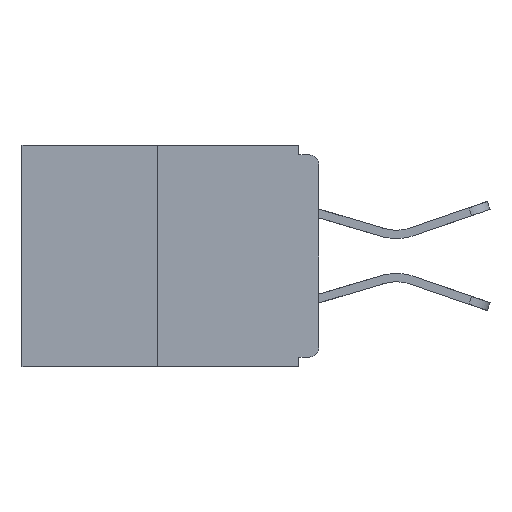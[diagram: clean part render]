
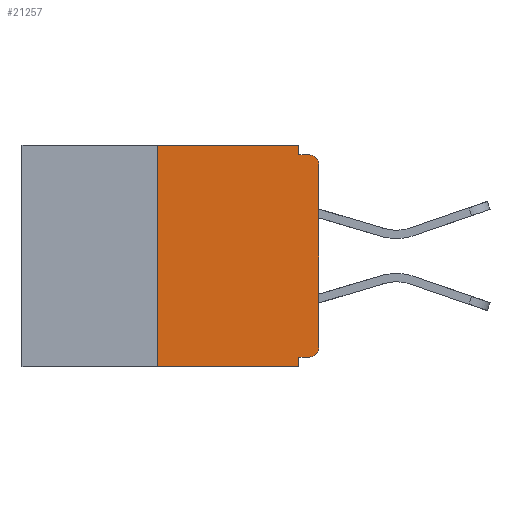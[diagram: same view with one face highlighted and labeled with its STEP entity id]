
A CAD part, left-side view. The second image highlights one B-rep face of the part: STEP entity #21257.
In plain terms, the highlighted planar face has unit normal (-1, 0, 0).
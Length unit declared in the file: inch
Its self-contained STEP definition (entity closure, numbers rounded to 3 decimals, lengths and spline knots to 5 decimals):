
#654 = CARTESIAN_POINT ( 'NONE',  ( 0., 0.031, 0. ) ) ;
#706 = DIRECTION ( 'NONE',  ( 0., 0., -1. ) ) ;
#2101 = CARTESIAN_POINT ( 'NONE',  ( 0., 0.25, -0.343 ) ) ;
#2222 = DIRECTION ( 'NONE',  ( 0., -1., 0. ) ) ;
#2345 = EDGE_LOOP ( 'NONE', ( #25715, #24356, #23364, #6456, #25840, #10254, #25453, #20279, #23910, #20800 ) ) ;
#2973 = CARTESIAN_POINT ( 'NONE',  ( 0., 0., 0. ) ) ;
#3060 = LINE ( 'NONE', #14448, #18005 ) ;
#3343 = CARTESIAN_POINT ( 'NONE',  ( 0., 0., -0.313 ) ) ;
#3421 = DIRECTION ( 'NONE',  ( -1., 0., 0. ) ) ;
#3853 = PLANE ( 'NONE',  #10965 ) ;
#4095 = FACE_OUTER_BOUND ( 'NONE', #2345, .T. ) ;
#4282 = CARTESIAN_POINT ( 'NONE',  ( 0., 0.015, -0.313 ) ) ;
#4431 = CARTESIAN_POINT ( 'NONE',  ( 0., 0., -0.328 ) ) ;
#4645 = CARTESIAN_POINT ( 'NONE',  ( 0., 0., -0.03 ) ) ;
#5353 = VERTEX_POINT ( 'NONE', #16338 ) ;
#6342 = DIRECTION ( 'NONE',  ( 0., 0., -1. ) ) ;
#6456 = ORIENTED_EDGE ( 'NONE', *, *, #26074, .F. ) ;
#6630 = CARTESIAN_POINT ( 'NONE',  ( 0., 0.46, -0.343 ) ) ;
#6662 = AXIS2_PLACEMENT_3D ( 'NONE', #15694, #3421, #9585 ) ;
#6745 = LINE ( 'NONE', #4431, #8318 ) ;
#6806 = VECTOR ( 'NONE', #12697, 39.37008 ) ;
#7884 = EDGE_CURVE ( 'NONE', #9522, #23636, #13813, .T. ) ;
#8318 = VECTOR ( 'NONE', #18672, 39.37008 ) ;
#8763 = CARTESIAN_POINT ( 'NONE',  ( 0., 0.015, -0.015 ) ) ;
#8769 = CARTESIAN_POINT ( 'NONE',  ( 0., 0.46, 0. ) ) ;
#9448 = CARTESIAN_POINT ( 'NONE',  ( 0., 0.031, -0.343 ) ) ;
#9522 = VERTEX_POINT ( 'NONE', #2101 ) ;
#9585 = DIRECTION ( 'NONE',  ( 0., 0., -1. ) ) ;
#9791 = EDGE_CURVE ( 'NONE', #18955, #23872, #25516, .T. ) ;
#9825 = DIRECTION ( 'NONE',  ( 0., 0., -1. ) ) ;
#9880 = EDGE_CURVE ( 'NONE', #17371, #15230, #22659, .T. ) ;
#10139 = LINE ( 'NONE', #17306, #19671 ) ;
#10254 = ORIENTED_EDGE ( 'NONE', *, *, #9880, .T. ) ;
#10605 = VERTEX_POINT ( 'NONE', #654 ) ;
#10965 = AXIS2_PLACEMENT_3D ( 'NONE', #15787, #22032, #19896 ) ;
#11363 = VERTEX_POINT ( 'NONE', #21166 ) ;
#11851 = VERTEX_POINT ( 'NONE', #20469 ) ;
#12511 = DIRECTION ( 'NONE',  ( -1., 0., 0. ) ) ;
#12588 = VECTOR ( 'NONE', #17211, 39.37008 ) ;
#12697 = DIRECTION ( 'NONE',  ( 0., -1., 0. ) ) ;
#13707 = LINE ( 'NONE', #13931, #24217 ) ;
#13813 = LINE ( 'NONE', #6630, #6806 ) ;
#13863 = LINE ( 'NONE', #2973, #12588 ) ;
#13931 = CARTESIAN_POINT ( 'NONE',  ( 0., 0.031, 0. ) ) ;
#14398 = LINE ( 'NONE', #25184, #21075 ) ;
#14448 = CARTESIAN_POINT ( 'NONE',  ( 0., 0., -0.015 ) ) ;
#15230 = VERTEX_POINT ( 'NONE', #3343 ) ;
#15578 = EDGE_CURVE ( 'NONE', #11363, #10605, #21980, .T. ) ;
#15694 = CARTESIAN_POINT ( 'NONE',  ( 0., 0.015, -0.03 ) ) ;
#15787 = CARTESIAN_POINT ( 'NONE',  ( 0., 0.46, 0. ) ) ;
#15808 = EDGE_CURVE ( 'NONE', #10605, #5353, #13707, .T. ) ;
#16338 = CARTESIAN_POINT ( 'NONE',  ( 0., 0.031, -0.015 ) ) ;
#16833 = DIRECTION ( 'NONE',  ( 0., -1., 0. ) ) ;
#17211 = DIRECTION ( 'NONE',  ( 0., 0., 1. ) ) ;
#17306 = CARTESIAN_POINT ( 'NONE',  ( 0., 0.25, 0. ) ) ;
#17371 = VERTEX_POINT ( 'NONE', #19542 ) ;
#17399 = AXIS2_PLACEMENT_3D ( 'NONE', #4282, #12511, #6342 ) ;
#17932 = EDGE_CURVE ( 'NONE', #15230, #18955, #13863, .T. ) ;
#18005 = VECTOR ( 'NONE', #2222, 39.37008 ) ;
#18672 = DIRECTION ( 'NONE',  ( 0., 1., 0. ) ) ;
#18955 = VERTEX_POINT ( 'NONE', #4645 ) ;
#19542 = CARTESIAN_POINT ( 'NONE',  ( 0., 0.015, -0.328 ) ) ;
#19671 = VECTOR ( 'NONE', #25588, 39.37008 ) ;
#19896 = DIRECTION ( 'NONE',  ( 0., 0., -1. ) ) ;
#20279 = ORIENTED_EDGE ( 'NONE', *, *, #9791, .T. ) ;
#20469 = CARTESIAN_POINT ( 'NONE',  ( 0., 0.031, -0.328 ) ) ;
#20800 = ORIENTED_EDGE ( 'NONE', *, *, #15808, .F. ) ;
#21075 = VECTOR ( 'NONE', #706, 39.37008 ) ;
#21166 = CARTESIAN_POINT ( 'NONE',  ( 0., 0.25, 0. ) ) ;
#21257 = ADVANCED_FACE ( 'NONE', ( #4095 ), #3853, .F. ) ;
#21857 = EDGE_CURVE ( 'NONE', #9522, #11363, #10139, .T. ) ;
#21980 = LINE ( 'NONE', #8769, #22642 ) ;
#22032 = DIRECTION ( 'NONE',  ( 1., 0., 0. ) ) ;
#22642 = VECTOR ( 'NONE', #16833, 39.37008 ) ;
#22659 = CIRCLE ( 'NONE', #17399, 0.015 ) ;
#23277 = EDGE_CURVE ( 'NONE', #5353, #23872, #3060, .T. ) ;
#23364 = ORIENTED_EDGE ( 'NONE', *, *, #7884, .T. ) ;
#23636 = VERTEX_POINT ( 'NONE', #9448 ) ;
#23872 = VERTEX_POINT ( 'NONE', #8763 ) ;
#23910 = ORIENTED_EDGE ( 'NONE', *, *, #23277, .F. ) ;
#24217 = VECTOR ( 'NONE', #9825, 39.37008 ) ;
#24356 = ORIENTED_EDGE ( 'NONE', *, *, #21857, .F. ) ;
#25184 = CARTESIAN_POINT ( 'NONE',  ( 0., 0.031, -0.343 ) ) ;
#25453 = ORIENTED_EDGE ( 'NONE', *, *, #17932, .T. ) ;
#25516 = CIRCLE ( 'NONE', #6662, 0.015 ) ;
#25588 = DIRECTION ( 'NONE',  ( 0., 0., 1. ) ) ;
#25715 = ORIENTED_EDGE ( 'NONE', *, *, #15578, .F. ) ;
#25840 = ORIENTED_EDGE ( 'NONE', *, *, #25969, .F. ) ;
#25969 = EDGE_CURVE ( 'NONE', #17371, #11851, #6745, .T. ) ;
#26074 = EDGE_CURVE ( 'NONE', #11851, #23636, #14398, .T. ) ;
